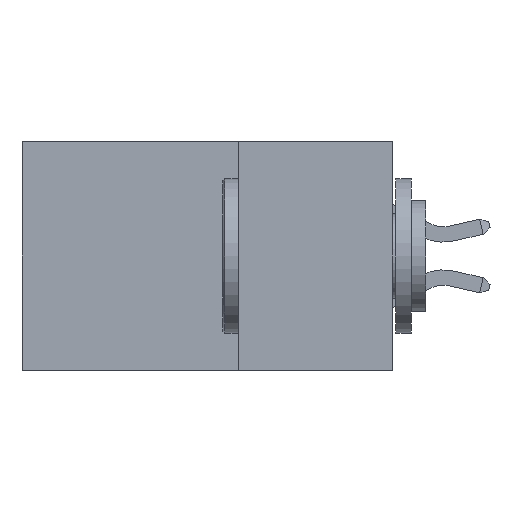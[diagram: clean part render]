
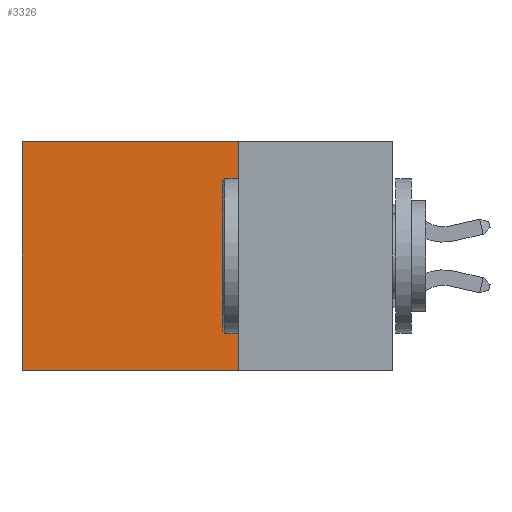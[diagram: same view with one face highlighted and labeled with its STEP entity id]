
A CAD part, left-side view. The second image highlights one B-rep face of the part: STEP entity #3326.
In plain terms, the highlighted planar face has unit normal (-1, 0, 0).
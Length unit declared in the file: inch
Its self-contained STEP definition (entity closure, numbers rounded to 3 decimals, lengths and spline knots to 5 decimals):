
#2200 = CARTESIAN_POINT ( 'NONE',  ( 0.2875, 0.6, 0. ) ) ;
#3179 = DIRECTION ( 'NONE',  ( 0., 1., 0. ) ) ;
#3326 = ADVANCED_FACE ( 'NONE', ( #17508 ), #8317, .F. ) ;
#3894 = VECTOR ( 'NONE', #21441, 39.37008 ) ;
#4279 = VERTEX_POINT ( 'NONE', #29578 ) ;
#4334 = CARTESIAN_POINT ( 'NONE',  ( 0.2875, 0.25, 0. ) ) ;
#5071 = CARTESIAN_POINT ( 'NONE',  ( 0.2875, 0.25, 0. ) ) ;
#7091 = VERTEX_POINT ( 'NONE', #34023 ) ;
#7094 = LINE ( 'NONE', #5071, #11366 ) ;
#7763 = ORIENTED_EDGE ( 'NONE', *, *, #29917, .F. ) ;
#7962 = VERTEX_POINT ( 'NONE', #4334 ) ;
#8317 = PLANE ( 'NONE',  #10402 ) ;
#8551 = VECTOR ( 'NONE', #9026, 39.37008 ) ;
#9026 = DIRECTION ( 'NONE',  ( 0., 1., 0. ) ) ;
#10402 = AXIS2_PLACEMENT_3D ( 'NONE', #19402, #30539, #22504 ) ;
#11366 = VECTOR ( 'NONE', #32502, 39.37008 ) ;
#13694 = LINE ( 'NONE', #16850, #21393 ) ;
#15801 = LINE ( 'NONE', #2200, #3894 ) ;
#16094 = ORIENTED_EDGE ( 'NONE', *, *, #26724, .F. ) ;
#16850 = CARTESIAN_POINT ( 'NONE',  ( 0.2875, 0.25, -0.37 ) ) ;
#17508 = FACE_OUTER_BOUND ( 'NONE', #32510, .T. ) ;
#19402 = CARTESIAN_POINT ( 'NONE',  ( 0.2875, 0.25, 0. ) ) ;
#19491 = EDGE_CURVE ( 'NONE', #7091, #4279, #15801, .T. ) ;
#19495 = VERTEX_POINT ( 'NONE', #29138 ) ;
#21393 = VECTOR ( 'NONE', #3179, 39.37008 ) ;
#21441 = DIRECTION ( 'NONE',  ( 0., 0., -1. ) ) ;
#22504 = DIRECTION ( 'NONE',  ( 0., 0., -1. ) ) ;
#23121 = ORIENTED_EDGE ( 'NONE', *, *, #19491, .T. ) ;
#25328 = CARTESIAN_POINT ( 'NONE',  ( 0.2875, 0.25, 0. ) ) ;
#26724 = EDGE_CURVE ( 'NONE', #7962, #19495, #7094, .T. ) ;
#29138 = CARTESIAN_POINT ( 'NONE',  ( 0.2875, 0.25, -0.37 ) ) ;
#29578 = CARTESIAN_POINT ( 'NONE',  ( 0.2875, 0.6, -0.37 ) ) ;
#29917 = EDGE_CURVE ( 'NONE', #19495, #4279, #13694, .T. ) ;
#30539 = DIRECTION ( 'NONE',  ( 1., 0., 0. ) ) ;
#32502 = DIRECTION ( 'NONE',  ( 0., 0., -1. ) ) ;
#32510 = EDGE_LOOP ( 'NONE', ( #23121, #7763, #16094, #34272 ) ) ;
#34023 = CARTESIAN_POINT ( 'NONE',  ( 0.2875, 0.6, 0. ) ) ;
#34272 = ORIENTED_EDGE ( 'NONE', *, *, #34809, .T. ) ;
#34498 = LINE ( 'NONE', #25328, #8551 ) ;
#34809 = EDGE_CURVE ( 'NONE', #7962, #7091, #34498, .T. ) ;
